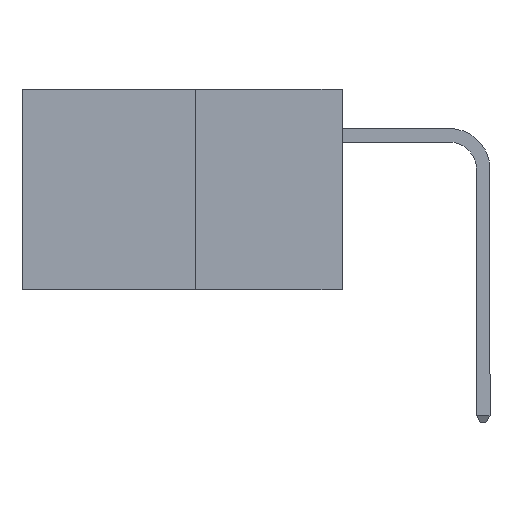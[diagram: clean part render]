
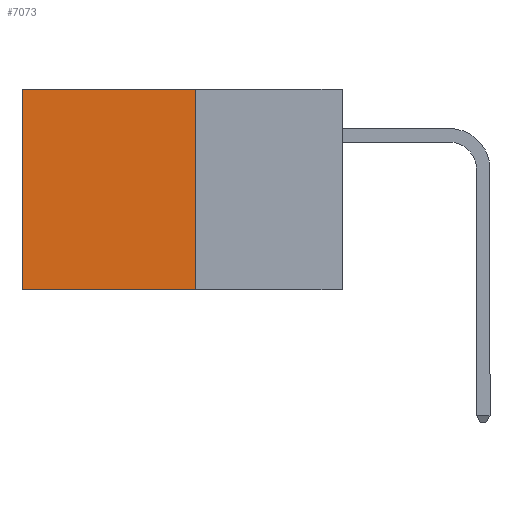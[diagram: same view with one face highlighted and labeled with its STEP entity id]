
A CAD part, left-side view. The second image highlights one B-rep face of the part: STEP entity #7073.
In plain terms, the highlighted planar face has unit normal (-1, 0, 0).
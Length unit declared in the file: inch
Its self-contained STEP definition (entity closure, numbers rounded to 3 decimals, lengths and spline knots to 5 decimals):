
#70 = ORIENTED_EDGE ( 'NONE', *, *, #3658, .F. ) ;
#241 = VECTOR ( 'NONE', #5113, 39.37008 ) ;
#1704 = EDGE_CURVE ( 'NONE', #10046, #9332, #2862, .T. ) ;
#2014 = DIRECTION ( 'NONE',  ( 1., 0., 0. ) ) ;
#2543 = CARTESIAN_POINT ( 'NONE',  ( 0.277, 0.27, -0.37 ) ) ;
#2862 = LINE ( 'NONE', #10074, #7873 ) ;
#2946 = LINE ( 'NONE', #2543, #3280 ) ;
#3023 = LINE ( 'NONE', #3044, #241 ) ;
#3044 = CARTESIAN_POINT ( 'NONE',  ( 0.277, 0.59, -0.37 ) ) ;
#3280 = VECTOR ( 'NONE', #3986, 39.37008 ) ;
#3651 = CARTESIAN_POINT ( 'NONE',  ( 0.277, 0.59, -0.37 ) ) ;
#3658 = EDGE_CURVE ( 'NONE', #10288, #4543, #11939, .T. ) ;
#3986 = DIRECTION ( 'NONE',  ( 0., 0., -1. ) ) ;
#4298 = VECTOR ( 'NONE', #8781, 39.37008 ) ;
#4352 = ORIENTED_EDGE ( 'NONE', *, *, #1704, .T. ) ;
#4543 = VERTEX_POINT ( 'NONE', #3651 ) ;
#4692 = EDGE_CURVE ( 'NONE', #10046, #10288, #2946, .T. ) ;
#4769 = AXIS2_PLACEMENT_3D ( 'NONE', #6102, #2014, #8995 ) ;
#5113 = DIRECTION ( 'NONE',  ( 0., 0., -1. ) ) ;
#6102 = CARTESIAN_POINT ( 'NONE',  ( 0.277, 0.27, -0.37 ) ) ;
#6471 = EDGE_LOOP ( 'NONE', ( #7850, #70, #9914, #4352 ) ) ;
#7073 = ADVANCED_FACE ( 'NONE', ( #8768 ), #8053, .F. ) ;
#7268 = CARTESIAN_POINT ( 'NONE',  ( 0.277, 0.59, 0. ) ) ;
#7850 = ORIENTED_EDGE ( 'NONE', *, *, #11735, .T. ) ;
#7873 = VECTOR ( 'NONE', #10066, 39.37008 ) ;
#7932 = CARTESIAN_POINT ( 'NONE',  ( 0.277, 0.27, 0. ) ) ;
#8053 = PLANE ( 'NONE',  #4769 ) ;
#8302 = CARTESIAN_POINT ( 'NONE',  ( 0.277, 0.27, -0.37 ) ) ;
#8768 = FACE_OUTER_BOUND ( 'NONE', #6471, .T. ) ;
#8781 = DIRECTION ( 'NONE',  ( 0., 1., 0. ) ) ;
#8995 = DIRECTION ( 'NONE',  ( 0., 0., -1. ) ) ;
#9332 = VERTEX_POINT ( 'NONE', #7268 ) ;
#9914 = ORIENTED_EDGE ( 'NONE', *, *, #4692, .F. ) ;
#10046 = VERTEX_POINT ( 'NONE', #7932 ) ;
#10066 = DIRECTION ( 'NONE',  ( 0., 1., 0. ) ) ;
#10074 = CARTESIAN_POINT ( 'NONE',  ( 0.277, 0.27, 0. ) ) ;
#10288 = VERTEX_POINT ( 'NONE', #8302 ) ;
#11735 = EDGE_CURVE ( 'NONE', #9332, #4543, #3023, .T. ) ;
#11787 = CARTESIAN_POINT ( 'NONE',  ( 0.277, 0.27, -0.37 ) ) ;
#11939 = LINE ( 'NONE', #11787, #4298 ) ;
